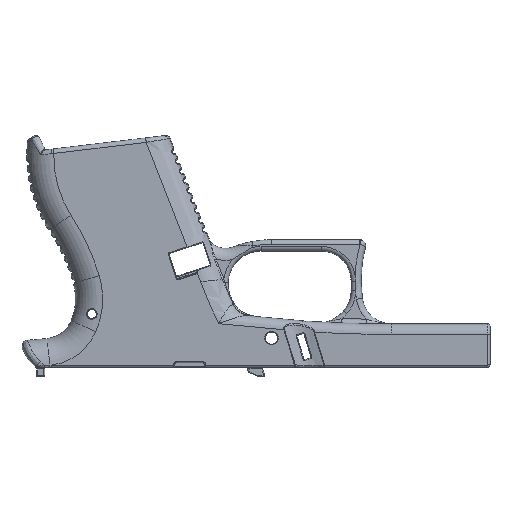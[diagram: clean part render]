
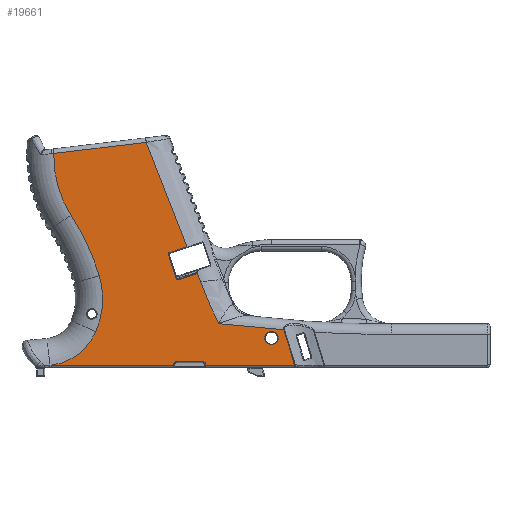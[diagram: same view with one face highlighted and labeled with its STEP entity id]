
A CAD part, front view. The second image highlights one B-rep face of the part: STEP entity #19661.
In plain terms, the highlighted planar face has unit normal (0, -1, 0).
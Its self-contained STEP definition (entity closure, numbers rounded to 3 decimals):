
#201=FACE_BOUND('',#5934,.T.);
#253=PLANE('',#21292);
#2242=LINE('',#32860,#3206);
#2245=LINE('',#32870,#3209);
#2249=LINE('',#32882,#3213);
#2264=LINE('',#33252,#3228);
#2265=LINE('',#33254,#3229);
#2266=LINE('',#33264,#3230);
#2267=LINE('',#33266,#3231);
#2268=LINE('',#33270,#3232);
#2269=LINE('',#33274,#3233);
#2270=LINE('',#33276,#3234);
#2271=LINE('',#33278,#3235);
#2272=LINE('',#33280,#3236);
#2273=LINE('',#33283,#3237);
#3206=VECTOR('',#24284,10.);
#3209=VECTOR('',#24295,10.);
#3213=VECTOR('',#24307,10.);
#3228=VECTOR('',#24330,10.);
#3229=VECTOR('',#24331,10.);
#3230=VECTOR('',#24340,10.);
#3231=VECTOR('',#24341,10.);
#3232=VECTOR('',#24344,10.);
#3233=VECTOR('',#24347,10.);
#3234=VECTOR('',#24348,10.);
#3235=VECTOR('',#24349,10.);
#3236=VECTOR('',#24350,10.);
#3237=VECTOR('',#24353,10.);
#4589=FACE_OUTER_BOUND('',#5933,.T.);
#5933=EDGE_LOOP('',(#14528,#14529,#14530,#14531,#14532,#14533,#14534,#14535,
#14536,#14537,#14538,#14539,#14540,#14541,#14542,#14543,#14544,#14545,#14546,
#14547,#14548,#14549,#14550));
#5934=EDGE_LOOP('',(#14551));
#7279=CIRCLE('',#21283,0.49);
#7281=CIRCLE('',#21287,0.49);
#7283=CIRCLE('',#21291,0.49);
#7284=CIRCLE('',#21293,35.645);
#7285=CIRCLE('',#21294,77.599);
#7286=CIRCLE('',#21295,27.167);
#7287=CIRCLE('',#21296,18.891);
#7288=CIRCLE('',#21297,0.8);
#7289=CIRCLE('',#21298,0.8);
#7290=CIRCLE('',#21299,156.771);
#7291=CIRCLE('',#21300,2.25);
#8700=VERTEX_POINT('',#32857);
#8701=VERTEX_POINT('',#32859);
#8702=VERTEX_POINT('',#32863);
#8704=VERTEX_POINT('',#32869);
#8706=VERTEX_POINT('',#32875);
#8708=VERTEX_POINT('',#32881);
#8710=VERTEX_POINT('',#32887);
#8730=VERTEX_POINT('',#33251);
#8731=VERTEX_POINT('',#33253);
#8732=VERTEX_POINT('',#33255);
#8733=VERTEX_POINT('',#33257);
#8734=VERTEX_POINT('',#33259);
#8735=VERTEX_POINT('',#33261);
#8736=VERTEX_POINT('',#33263);
#8737=VERTEX_POINT('',#33265);
#8738=VERTEX_POINT('',#33267);
#8739=VERTEX_POINT('',#33269);
#8740=VERTEX_POINT('',#33271);
#8741=VERTEX_POINT('',#33273);
#8742=VERTEX_POINT('',#33275);
#8743=VERTEX_POINT('',#33277);
#8744=VERTEX_POINT('',#33279);
#8745=VERTEX_POINT('',#33281);
#8746=VERTEX_POINT('',#33284);
#10775=EDGE_CURVE('',#8700,#8701,#2242,.T.);
#10779=EDGE_CURVE('',#8701,#8702,#7279,.T.);
#10780=EDGE_CURVE('',#8702,#8704,#2245,.T.);
#10785=EDGE_CURVE('',#8704,#8706,#7281,.T.);
#10786=EDGE_CURVE('',#8706,#8708,#2249,.T.);
#10791=EDGE_CURVE('',#8708,#8710,#7283,.T.);
#10825=EDGE_CURVE('',#8700,#8730,#2264,.T.);
#10826=EDGE_CURVE('',#8731,#8730,#2265,.T.);
#10827=EDGE_CURVE('',#8732,#8731,#7284,.T.);
#10828=EDGE_CURVE('',#8733,#8732,#7285,.T.);
#10829=EDGE_CURVE('',#8734,#8733,#7286,.T.);
#10830=EDGE_CURVE('',#8735,#8734,#7287,.T.);
#10831=EDGE_CURVE('',#8736,#8735,#2266,.T.);
#10832=EDGE_CURVE('',#8737,#8736,#2267,.T.);
#10833=EDGE_CURVE('',#8738,#8737,#7288,.T.);
#10834=EDGE_CURVE('',#8739,#8738,#2268,.T.);
#10835=EDGE_CURVE('',#8740,#8739,#7289,.T.);
#10836=EDGE_CURVE('',#8741,#8740,#2269,.T.);
#10837=EDGE_CURVE('',#8742,#8741,#2270,.T.);
#10838=EDGE_CURVE('',#8743,#8742,#2271,.T.);
#10839=EDGE_CURVE('',#8744,#8743,#2272,.T.);
#10840=EDGE_CURVE('',#8745,#8744,#7290,.T.);
#10841=EDGE_CURVE('',#8745,#8710,#2273,.T.);
#10842=EDGE_CURVE('',#8746,#8746,#7291,.T.);
#14528=ORIENTED_EDGE('',*,*,#10791,.F.);
#14529=ORIENTED_EDGE('',*,*,#10786,.F.);
#14530=ORIENTED_EDGE('',*,*,#10785,.F.);
#14531=ORIENTED_EDGE('',*,*,#10780,.F.);
#14532=ORIENTED_EDGE('',*,*,#10779,.F.);
#14533=ORIENTED_EDGE('',*,*,#10775,.F.);
#14534=ORIENTED_EDGE('',*,*,#10825,.T.);
#14535=ORIENTED_EDGE('',*,*,#10826,.F.);
#14536=ORIENTED_EDGE('',*,*,#10827,.F.);
#14537=ORIENTED_EDGE('',*,*,#10828,.F.);
#14538=ORIENTED_EDGE('',*,*,#10829,.F.);
#14539=ORIENTED_EDGE('',*,*,#10830,.F.);
#14540=ORIENTED_EDGE('',*,*,#10831,.F.);
#14541=ORIENTED_EDGE('',*,*,#10832,.F.);
#14542=ORIENTED_EDGE('',*,*,#10833,.F.);
#14543=ORIENTED_EDGE('',*,*,#10834,.F.);
#14544=ORIENTED_EDGE('',*,*,#10835,.F.);
#14545=ORIENTED_EDGE('',*,*,#10836,.F.);
#14546=ORIENTED_EDGE('',*,*,#10837,.F.);
#14547=ORIENTED_EDGE('',*,*,#10838,.F.);
#14548=ORIENTED_EDGE('',*,*,#10839,.F.);
#14549=ORIENTED_EDGE('',*,*,#10840,.F.);
#14550=ORIENTED_EDGE('',*,*,#10841,.T.);
#14551=ORIENTED_EDGE('',*,*,#10842,.F.);
#19661=ADVANCED_FACE('',(#4589,#201),#253,.F.);
#21283=AXIS2_PLACEMENT_3D('',#32867,#24291,#24292);
#21287=AXIS2_PLACEMENT_3D('',#32879,#24303,#24304);
#21291=AXIS2_PLACEMENT_3D('',#32891,#24315,#24316);
#21292=AXIS2_PLACEMENT_3D('',#33250,#24328,#24329);
#21293=AXIS2_PLACEMENT_3D('',#33256,#24332,#24333);
#21294=AXIS2_PLACEMENT_3D('',#33258,#24334,#24335);
#21295=AXIS2_PLACEMENT_3D('',#33260,#24336,#24337);
#21296=AXIS2_PLACEMENT_3D('',#33262,#24338,#24339);
#21297=AXIS2_PLACEMENT_3D('',#33268,#24342,#24343);
#21298=AXIS2_PLACEMENT_3D('',#33272,#24345,#24346);
#21299=AXIS2_PLACEMENT_3D('',#33282,#24351,#24352);
#21300=AXIS2_PLACEMENT_3D('',#33285,#24354,#24355);
#24284=DIRECTION('',(-0.951,0.,-0.309));
#24291=DIRECTION('center_axis',(0.,-1.,0.));
#24292=DIRECTION('ref_axis',(-0.891,0.,0.454));
#24295=DIRECTION('',(0.309,0.,-0.951));
#24303=DIRECTION('center_axis',(0.,-1.,0.));
#24304=DIRECTION('ref_axis',(-0.454,0.,-0.891));
#24307=DIRECTION('',(0.951,0.,0.309));
#24315=DIRECTION('center_axis',(0.,-1.,0.));
#24316=DIRECTION('ref_axis',(0.891,0.,-0.454));
#24328=DIRECTION('center_axis',(0.,1.,0.));
#24329=DIRECTION('ref_axis',(1.,0.,0.));
#24330=DIRECTION('',(-0.363,0.,0.932));
#24331=DIRECTION('',(0.993,0.,0.119));
#24332=DIRECTION('center_axis',(0.,1.,0.));
#24333=DIRECTION('ref_axis',(-0.961,0.,-0.276));
#24334=DIRECTION('center_axis',(0.,-1.,0.));
#24335=DIRECTION('ref_axis',(0.907,0.,0.421));
#24336=DIRECTION('center_axis',(0.,-1.,0.));
#24337=DIRECTION('ref_axis',(0.998,0.,-0.06));
#24338=DIRECTION('center_axis',(0.,-1.,0.));
#24339=DIRECTION('ref_axis',(0.592,0.,-0.806));
#24340=DIRECTION('',(-1.,0.,0.));
#24341=DIRECTION('',(0.,0.,-1.));
#24342=DIRECTION('center_axis',(0.,-1.,0.));
#24343=DIRECTION('ref_axis',(-0.707,0.,0.707));
#24344=DIRECTION('',(-1.,0.,0.));
#24345=DIRECTION('center_axis',(0.,-1.,0.));
#24346=DIRECTION('ref_axis',(0.707,0.,0.707));
#24347=DIRECTION('',(0.,0.,1.));
#24348=DIRECTION('',(-1.,0.,0.));
#24349=DIRECTION('',(0.292,0.,-0.956));
#24350=DIRECTION('',(0.996,0.,-0.092));
#24351=DIRECTION('center_axis',(0.,-1.,0.));
#24352=DIRECTION('ref_axis',(-0.937,0.,-0.35));
#24353=DIRECTION('',(-0.363,0.,0.932));
#24354=DIRECTION('center_axis',(0.,-1.,0.));
#24355=DIRECTION('ref_axis',(1.,0.,0.));
#32857=CARTESIAN_POINT('',(-24.666,-11.5,13.614));
#32859=CARTESIAN_POINT('',(-30.54,-11.5,11.706));
#32860=CARTESIAN_POINT('',(-17.775,-11.5,15.853));
#32863=CARTESIAN_POINT('',(-30.854,-11.5,11.088));
#32867=CARTESIAN_POINT('Origin',(-30.388,-11.5,11.24));
#32869=CARTESIAN_POINT('',(-28.228,-11.5,3.004));
#32870=CARTESIAN_POINT('',(-28.236,-11.5,3.028));
#32875=CARTESIAN_POINT('',(-27.61,-11.5,2.69));
#32879=CARTESIAN_POINT('Origin',(-27.762,-11.5,3.156));
#32881=CARTESIAN_POINT('',(-21.428,-11.5,4.698));
#32882=CARTESIAN_POINT('',(-11.516,-11.5,7.919));
#32887=CARTESIAN_POINT('',(-21.238,-11.5,4.813));
#32891=CARTESIAN_POINT('Origin',(-21.58,-11.5,5.164));
#33250=CARTESIAN_POINT('Origin',(-1.777,-11.5,10.863));
#33251=CARTESIAN_POINT('',(-38.228,-11.5,48.431));
#33252=CARTESIAN_POINT('',(-37.545,-11.5,46.678));
#33253=CARTESIAN_POINT('',(-68.991,-11.5,44.75));
#33254=CARTESIAN_POINT('',(-18.413,-11.5,50.802));
#33255=CARTESIAN_POINT('',(-63.213,-11.5,24.169));
#33256=CARTESIAN_POINT('Origin',(-33.363,-11.5,43.651));
#33257=CARTESIAN_POINT('',(-53.881,-11.5,4.09));
#33258=CARTESIAN_POINT('Origin',(-128.196,-11.5,-18.243));
#33259=CARTESIAN_POINT('',(-55.002,-11.5,-14.602));
#33260=CARTESIAN_POINT('Origin',(-79.899,-11.5,-3.729));
#33261=CARTESIAN_POINT('',(-69.695,-11.5,-25.75));
#33262=CARTESIAN_POINT('Origin',(-72.315,-11.5,-7.041));
#33263=CARTESIAN_POINT('',(-29.05,-11.5,-25.75));
#33264=CARTESIAN_POINT('',(37.236,-11.5,-25.75));
#33265=CARTESIAN_POINT('',(-29.05,-11.5,-25.475));
#33266=CARTESIAN_POINT('',(-29.05,-11.5,-7.056));
#33267=CARTESIAN_POINT('',(-28.25,-11.5,-24.675));
#33268=CARTESIAN_POINT('Origin',(-28.25,-11.5,-25.475));
#33269=CARTESIAN_POINT('',(-19.25,-11.5,-24.675));
#33270=CARTESIAN_POINT('',(-10.264,-11.5,-24.675));
#33271=CARTESIAN_POINT('',(-18.45,-11.5,-25.475));
#33272=CARTESIAN_POINT('Origin',(-19.25,-11.5,-25.475));
#33273=CARTESIAN_POINT('',(-18.45,-11.5,-25.75));
#33274=CARTESIAN_POINT('',(-18.45,-11.5,-7.818));
#33275=CARTESIAN_POINT('',(11.185,-11.5,-25.75));
#33276=CARTESIAN_POINT('',(37.236,-11.5,-25.75));
#33277=CARTESIAN_POINT('',(7.57,-11.5,-13.924));
#33278=CARTESIAN_POINT('',(5.553,-11.5,-7.328));
#33279=CARTESIAN_POINT('',(-14.141,-11.5,-11.929));
#33280=CARTESIAN_POINT('',(4.861,-11.5,-13.675));
#33281=CARTESIAN_POINT('',(-20.166,-11.5,2.06));
#33282=CARTESIAN_POINT('Origin',(126.663,-11.5,57.001));
#33283=CARTESIAN_POINT('',(-37.545,-11.5,46.678));
#33284=CARTESIAN_POINT('',(1.25,-11.5,-16.75));
#33285=CARTESIAN_POINT('Origin',(3.5,-11.5,-16.75));
